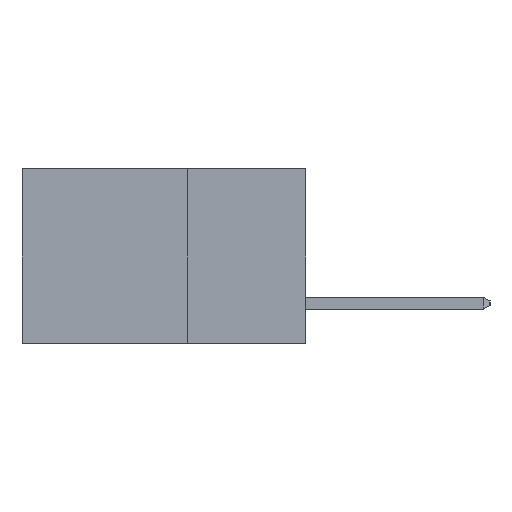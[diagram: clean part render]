
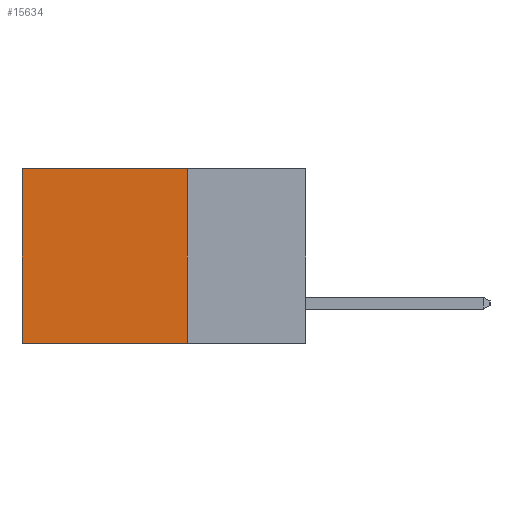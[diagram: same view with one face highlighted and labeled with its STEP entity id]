
A CAD part, left-side view. The second image highlights one B-rep face of the part: STEP entity #15634.
In plain terms, the highlighted planar face has unit normal (-1, 0, 0).
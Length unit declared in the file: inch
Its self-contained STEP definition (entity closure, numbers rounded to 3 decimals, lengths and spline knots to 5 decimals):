
#198 = ORIENTED_EDGE ( 'NONE', *, *, #5398, .T. ) ;
#1304 = EDGE_CURVE ( 'NONE', #2592, #5779, #17423, .T. ) ;
#1755 = CARTESIAN_POINT ( 'NONE',  ( 0.2615, 0.25, -0.37 ) ) ;
#2592 = VERTEX_POINT ( 'NONE', #22255 ) ;
#2822 = LINE ( 'NONE', #13325, #12442 ) ;
#3727 = DIRECTION ( 'NONE',  ( 0., 0., -1. ) ) ;
#3814 = DIRECTION ( 'NONE',  ( 0., 1., 0. ) ) ;
#5113 = EDGE_CURVE ( 'NONE', #2592, #9794, #7280, .T. ) ;
#5364 = DIRECTION ( 'NONE',  ( 0., 0., -1. ) ) ;
#5398 = EDGE_CURVE ( 'NONE', #5779, #19039, #10892, .T. ) ;
#5733 = EDGE_LOOP ( 'NONE', ( #198, #18584, #21388, #23215 ) ) ;
#5779 = VERTEX_POINT ( 'NONE', #13705 ) ;
#5859 = CARTESIAN_POINT ( 'NONE',  ( 0.2615, 0.25, -0.37 ) ) ;
#7280 = LINE ( 'NONE', #5859, #21521 ) ;
#7410 = VECTOR ( 'NONE', #8378, 39.37008 ) ;
#8378 = DIRECTION ( 'NONE',  ( 0., 1., 0. ) ) ;
#9343 = CARTESIAN_POINT ( 'NONE',  ( 0.2615, 0.6, -0.37 ) ) ;
#9794 = VERTEX_POINT ( 'NONE', #22628 ) ;
#10892 = LINE ( 'NONE', #9343, #15225 ) ;
#12442 = VECTOR ( 'NONE', #3814, 39.37008 ) ;
#13217 = AXIS2_PLACEMENT_3D ( 'NONE', #1755, #15117, #3727 ) ;
#13325 = CARTESIAN_POINT ( 'NONE',  ( 0.2615, 0.25, -0.37 ) ) ;
#13705 = CARTESIAN_POINT ( 'NONE',  ( 0.2615, 0.6, 0. ) ) ;
#15117 = DIRECTION ( 'NONE',  ( 1., 0., 0. ) ) ;
#15225 = VECTOR ( 'NONE', #20446, 39.37008 ) ;
#15634 = ADVANCED_FACE ( 'NONE', ( #21558 ), #22349, .F. ) ;
#17423 = LINE ( 'NONE', #19160, #7410 ) ;
#17522 = EDGE_CURVE ( 'NONE', #9794, #19039, #2822, .T. ) ;
#18584 = ORIENTED_EDGE ( 'NONE', *, *, #17522, .F. ) ;
#19039 = VERTEX_POINT ( 'NONE', #20193 ) ;
#19160 = CARTESIAN_POINT ( 'NONE',  ( 0.2615, 0.25, 0. ) ) ;
#20193 = CARTESIAN_POINT ( 'NONE',  ( 0.2615, 0.6, -0.37 ) ) ;
#20446 = DIRECTION ( 'NONE',  ( 0., 0., -1. ) ) ;
#21388 = ORIENTED_EDGE ( 'NONE', *, *, #5113, .F. ) ;
#21521 = VECTOR ( 'NONE', #5364, 39.37008 ) ;
#21558 = FACE_OUTER_BOUND ( 'NONE', #5733, .T. ) ;
#22255 = CARTESIAN_POINT ( 'NONE',  ( 0.2615, 0.25, 0. ) ) ;
#22349 = PLANE ( 'NONE',  #13217 ) ;
#22628 = CARTESIAN_POINT ( 'NONE',  ( 0.2615, 0.25, -0.37 ) ) ;
#23215 = ORIENTED_EDGE ( 'NONE', *, *, #1304, .T. ) ;
